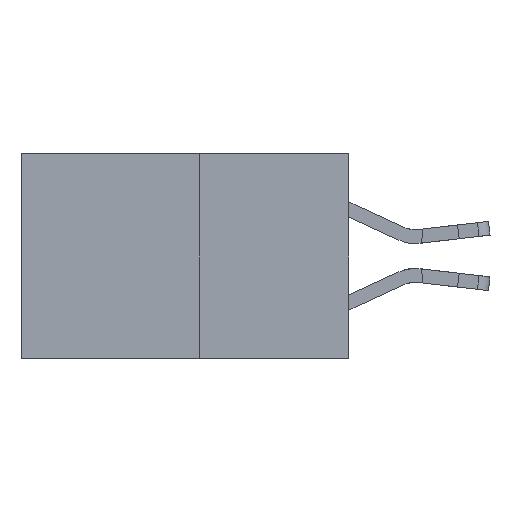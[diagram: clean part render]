
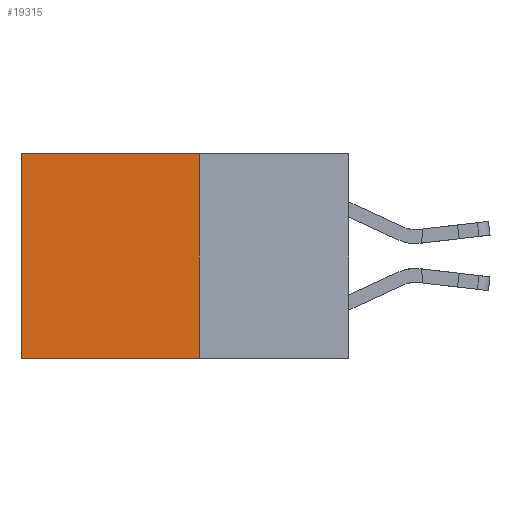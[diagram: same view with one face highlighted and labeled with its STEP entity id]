
A CAD part, left-side view. The second image highlights one B-rep face of the part: STEP entity #19315.
In plain terms, the highlighted planar face has unit normal (-1, 0, 0).
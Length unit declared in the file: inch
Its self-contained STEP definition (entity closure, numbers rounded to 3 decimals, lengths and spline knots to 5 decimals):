
#14 = VECTOR ( 'NONE', #951, 39.37008 ) ;
#951 = DIRECTION ( 'NONE',  ( 0., 0., -1. ) ) ;
#1624 = ORIENTED_EDGE ( 'NONE', *, *, #23578, .T. ) ;
#1695 = VERTEX_POINT ( 'NONE', #4405 ) ;
#2313 = LINE ( 'NONE', #7123, #16688 ) ;
#3401 = FACE_OUTER_BOUND ( 'NONE', #14730, .T. ) ;
#3966 = CARTESIAN_POINT ( 'NONE',  ( 0.277, 0.27, -0.37 ) ) ;
#4405 = CARTESIAN_POINT ( 'NONE',  ( 0.277, 0.59, 0. ) ) ;
#4870 = ORIENTED_EDGE ( 'NONE', *, *, #9280, .F. ) ;
#4938 = CARTESIAN_POINT ( 'NONE',  ( 0.277, 0.59, -0.37 ) ) ;
#5286 = ORIENTED_EDGE ( 'NONE', *, *, #21698, .F. ) ;
#5937 = DIRECTION ( 'NONE',  ( 0., 0., -1. ) ) ;
#7040 = DIRECTION ( 'NONE',  ( 0., 1., 0. ) ) ;
#7123 = CARTESIAN_POINT ( 'NONE',  ( 0.277, 0.27, -0.37 ) ) ;
#7467 = VERTEX_POINT ( 'NONE', #12544 ) ;
#7895 = VECTOR ( 'NONE', #24095, 39.37008 ) ;
#8139 = VERTEX_POINT ( 'NONE', #4938 ) ;
#9280 = EDGE_CURVE ( 'NONE', #18089, #8139, #2313, .T. ) ;
#9322 = PLANE ( 'NONE',  #15857 ) ;
#9750 = CARTESIAN_POINT ( 'NONE',  ( 0.277, 0.59, -0.37 ) ) ;
#10172 = LINE ( 'NONE', #12199, #14 ) ;
#11565 = DIRECTION ( 'NONE',  ( 0., 0., -1. ) ) ;
#12076 = LINE ( 'NONE', #9750, #20727 ) ;
#12199 = CARTESIAN_POINT ( 'NONE',  ( 0.277, 0.27, -0.37 ) ) ;
#12383 = EDGE_CURVE ( 'NONE', #7467, #1695, #18280, .T. ) ;
#12544 = CARTESIAN_POINT ( 'NONE',  ( 0.277, 0.27, 0. ) ) ;
#13111 = CARTESIAN_POINT ( 'NONE',  ( 0.277, 0.27, 0. ) ) ;
#14730 = EDGE_LOOP ( 'NONE', ( #1624, #4870, #5286, #17467 ) ) ;
#15857 = AXIS2_PLACEMENT_3D ( 'NONE', #3966, #17029, #5937 ) ;
#16688 = VECTOR ( 'NONE', #7040, 39.37008 ) ;
#17029 = DIRECTION ( 'NONE',  ( 1., 0., 0. ) ) ;
#17467 = ORIENTED_EDGE ( 'NONE', *, *, #12383, .T. ) ;
#18089 = VERTEX_POINT ( 'NONE', #23354 ) ;
#18280 = LINE ( 'NONE', #13111, #7895 ) ;
#19315 = ADVANCED_FACE ( 'NONE', ( #3401 ), #9322, .F. ) ;
#20727 = VECTOR ( 'NONE', #11565, 39.37008 ) ;
#21698 = EDGE_CURVE ( 'NONE', #7467, #18089, #10172, .T. ) ;
#23354 = CARTESIAN_POINT ( 'NONE',  ( 0.277, 0.27, -0.37 ) ) ;
#23578 = EDGE_CURVE ( 'NONE', #1695, #8139, #12076, .T. ) ;
#24095 = DIRECTION ( 'NONE',  ( 0., 1., 0. ) ) ;
